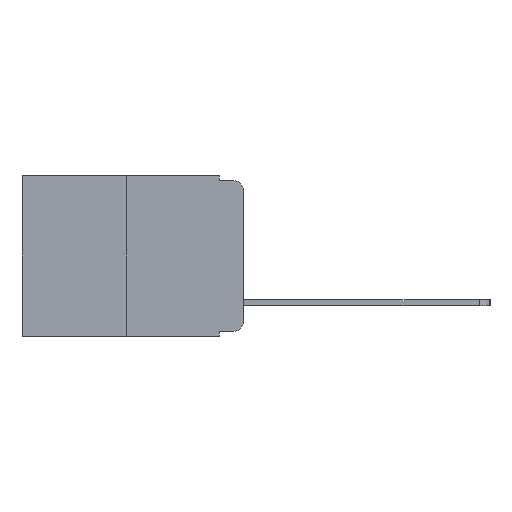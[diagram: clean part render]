
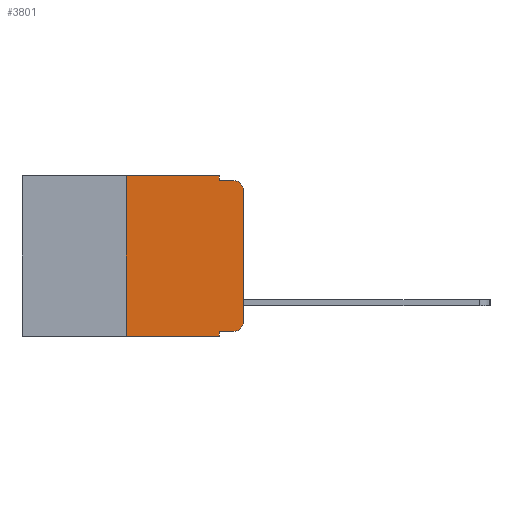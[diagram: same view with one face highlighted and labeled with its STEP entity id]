
A CAD part, left-side view. The second image highlights one B-rep face of the part: STEP entity #3801.
In plain terms, the highlighted planar face has unit normal (-1, 0, 0).
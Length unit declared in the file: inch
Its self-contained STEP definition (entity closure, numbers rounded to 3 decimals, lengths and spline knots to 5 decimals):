
#46 = CARTESIAN_POINT ( 'NONE',  ( 0., 0., -0.313 ) ) ;
#133 = CARTESIAN_POINT ( 'NONE',  ( 0., 0.473, -0.343 ) ) ;
#309 = VECTOR ( 'NONE', #14601, 39.37008 ) ;
#483 = CIRCLE ( 'NONE', #16887, 0.02 ) ;
#602 = CARTESIAN_POINT ( 'NONE',  ( 0., 0.051, -0.333 ) ) ;
#700 = DIRECTION ( 'NONE',  ( 0., -1., 0. ) ) ;
#742 = EDGE_CURVE ( 'NONE', #16759, #3595, #11436, .T. ) ;
#823 = ORIENTED_EDGE ( 'NONE', *, *, #8362, .T. ) ;
#1354 = EDGE_LOOP ( 'NONE', ( #1494, #16398, #10107, #4785, #12618, #17446, #2451, #2939, #823, #5289 ) ) ;
#1369 = CARTESIAN_POINT ( 'NONE',  ( 0., 0.473, 0. ) ) ;
#1415 = VECTOR ( 'NONE', #13586, 39.37008 ) ;
#1494 = ORIENTED_EDGE ( 'NONE', *, *, #7956, .T. ) ;
#1883 = LINE ( 'NONE', #14917, #1415 ) ;
#2147 = CARTESIAN_POINT ( 'NONE',  ( 0., 0.02, -0.03 ) ) ;
#2257 = CARTESIAN_POINT ( 'NONE',  ( 0., 0.051, 0. ) ) ;
#2328 = EDGE_CURVE ( 'NONE', #10456, #4836, #9094, .T. ) ;
#2362 = CARTESIAN_POINT ( 'NONE',  ( 0., 0.02, -0.313 ) ) ;
#2451 = ORIENTED_EDGE ( 'NONE', *, *, #2328, .T. ) ;
#2939 = ORIENTED_EDGE ( 'NONE', *, *, #11099, .F. ) ;
#2964 = CARTESIAN_POINT ( 'NONE',  ( 0., 0.02, -0.333 ) ) ;
#3265 = DIRECTION ( 'NONE',  ( 0., -1., 0. ) ) ;
#3595 = VERTEX_POINT ( 'NONE', #17266 ) ;
#3661 = DIRECTION ( 'NONE',  ( 0., 0., -1. ) ) ;
#3801 = ADVANCED_FACE ( 'NONE', ( #6710 ), #4341, .F. ) ;
#3865 = DIRECTION ( 'NONE',  ( 0., 0., -1. ) ) ;
#3939 = LINE ( 'NONE', #2257, #14199 ) ;
#3940 = CARTESIAN_POINT ( 'NONE',  ( 0., 0.051, -0.01 ) ) ;
#4234 = VECTOR ( 'NONE', #16566, 39.37008 ) ;
#4341 = PLANE ( 'NONE',  #15729 ) ;
#4785 = ORIENTED_EDGE ( 'NONE', *, *, #15115, .F. ) ;
#4836 = VERTEX_POINT ( 'NONE', #11465 ) ;
#5289 = ORIENTED_EDGE ( 'NONE', *, *, #16587, .T. ) ;
#5923 = VERTEX_POINT ( 'NONE', #2964 ) ;
#6334 = LINE ( 'NONE', #14448, #12730 ) ;
#6535 = VERTEX_POINT ( 'NONE', #16941 ) ;
#6710 = FACE_OUTER_BOUND ( 'NONE', #1354, .T. ) ;
#7848 = CARTESIAN_POINT ( 'NONE',  ( 0., 0.25, 0. ) ) ;
#7956 = EDGE_CURVE ( 'NONE', #17261, #15796, #1883, .T. ) ;
#8084 = CARTESIAN_POINT ( 'NONE',  ( 0., 0.02, -0.01 ) ) ;
#8182 = CARTESIAN_POINT ( 'NONE',  ( 0., 0.25, -0.343 ) ) ;
#8362 = EDGE_CURVE ( 'NONE', #11676, #5923, #6334, .T. ) ;
#8541 = LINE ( 'NONE', #14234, #4234 ) ;
#8593 = LINE ( 'NONE', #7848, #309 ) ;
#9094 = LINE ( 'NONE', #133, #12249 ) ;
#9809 = VECTOR ( 'NONE', #15034, 39.37008 ) ;
#9830 = EDGE_CURVE ( 'NONE', #6535, #14884, #13391, .T. ) ;
#10107 = ORIENTED_EDGE ( 'NONE', *, *, #9830, .F. ) ;
#10456 = VERTEX_POINT ( 'NONE', #8182 ) ;
#10494 = CARTESIAN_POINT ( 'NONE',  ( 0., 0., -0.03 ) ) ;
#10908 = DIRECTION ( 'NONE',  ( 0., 0., -1. ) ) ;
#11019 = VECTOR ( 'NONE', #12200, 39.37008 ) ;
#11099 = EDGE_CURVE ( 'NONE', #11676, #4836, #3939, .T. ) ;
#11436 = LINE ( 'NONE', #1369, #11019 ) ;
#11465 = CARTESIAN_POINT ( 'NONE',  ( 0., 0.051, -0.343 ) ) ;
#11657 = AXIS2_PLACEMENT_3D ( 'NONE', #2362, #12288, #3865 ) ;
#11676 = VERTEX_POINT ( 'NONE', #602 ) ;
#12111 = DIRECTION ( 'NONE',  ( -1., 0., 0. ) ) ;
#12200 = DIRECTION ( 'NONE',  ( 0., -1., 0. ) ) ;
#12249 = VECTOR ( 'NONE', #700, 39.37008 ) ;
#12288 = DIRECTION ( 'NONE',  ( -1., 0., 0. ) ) ;
#12618 = ORIENTED_EDGE ( 'NONE', *, *, #742, .F. ) ;
#12730 = VECTOR ( 'NONE', #3265, 39.37008 ) ;
#13391 = LINE ( 'NONE', #3940, #9809 ) ;
#13579 = EDGE_CURVE ( 'NONE', #10456, #16759, #8593, .T. ) ;
#13586 = DIRECTION ( 'NONE',  ( 0., 0., 1. ) ) ;
#14199 = VECTOR ( 'NONE', #10908, 39.37008 ) ;
#14234 = CARTESIAN_POINT ( 'NONE',  ( 0., 0.051, 0. ) ) ;
#14448 = CARTESIAN_POINT ( 'NONE',  ( 0., 0.051, -0.333 ) ) ;
#14601 = DIRECTION ( 'NONE',  ( 0., 0., 1. ) ) ;
#14875 = DIRECTION ( 'NONE',  ( 1., 0., 0. ) ) ;
#14884 = VERTEX_POINT ( 'NONE', #8084 ) ;
#14917 = CARTESIAN_POINT ( 'NONE',  ( 0., 0., 0. ) ) ;
#15034 = DIRECTION ( 'NONE',  ( 0., -1., 0. ) ) ;
#15115 = EDGE_CURVE ( 'NONE', #3595, #6535, #8541, .T. ) ;
#15310 = EDGE_CURVE ( 'NONE', #15796, #14884, #483, .T. ) ;
#15729 = AXIS2_PLACEMENT_3D ( 'NONE', #16584, #14875, #16581 ) ;
#15796 = VERTEX_POINT ( 'NONE', #10494 ) ;
#16398 = ORIENTED_EDGE ( 'NONE', *, *, #15310, .T. ) ;
#16448 = CIRCLE ( 'NONE', #11657, 0.02 ) ;
#16566 = DIRECTION ( 'NONE',  ( 0., 0., -1. ) ) ;
#16581 = DIRECTION ( 'NONE',  ( 0., 0., -1. ) ) ;
#16584 = CARTESIAN_POINT ( 'NONE',  ( 0., 0.473, 0. ) ) ;
#16587 = EDGE_CURVE ( 'NONE', #5923, #17261, #16448, .T. ) ;
#16722 = CARTESIAN_POINT ( 'NONE',  ( 0., 0.25, 0. ) ) ;
#16759 = VERTEX_POINT ( 'NONE', #16722 ) ;
#16887 = AXIS2_PLACEMENT_3D ( 'NONE', #2147, #12111, #3661 ) ;
#16941 = CARTESIAN_POINT ( 'NONE',  ( 0., 0.051, -0.01 ) ) ;
#17261 = VERTEX_POINT ( 'NONE', #46 ) ;
#17266 = CARTESIAN_POINT ( 'NONE',  ( 0., 0.051, 0. ) ) ;
#17446 = ORIENTED_EDGE ( 'NONE', *, *, #13579, .F. ) ;
